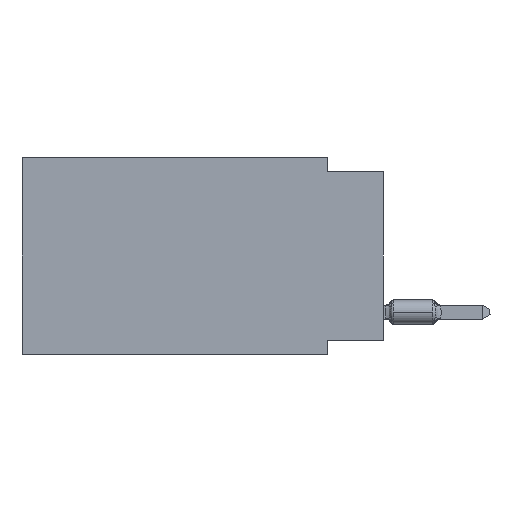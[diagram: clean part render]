
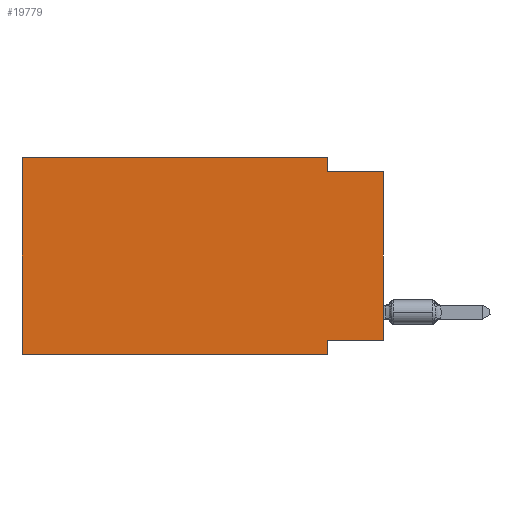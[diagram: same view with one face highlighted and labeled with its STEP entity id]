
A CAD part, left-side view. The second image highlights one B-rep face of the part: STEP entity #19779.
In plain terms, the highlighted planar face has unit normal (-1, 0, 0).
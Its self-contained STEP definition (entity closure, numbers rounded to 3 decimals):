
#254 = CARTESIAN_POINT ( 'NONE',  ( 0., 0., -0.635 ) ) ;
#355 = PLANE ( 'NONE',  #38991 ) ;
#422 = EDGE_CURVE ( 'NONE', #14213, #34933, #4034, .T. ) ;
#1116 = ORIENTED_EDGE ( 'NONE', *, *, #2686, .T. ) ;
#1243 = VECTOR ( 'NONE', #6488, 1000. ) ;
#1338 = EDGE_CURVE ( 'NONE', #21616, #13241, #23218, .T. ) ;
#1912 = VECTOR ( 'NONE', #14163, 1000. ) ;
#2667 = CARTESIAN_POINT ( 'NONE',  ( 0., 16.383, 0. ) ) ;
#2686 = EDGE_CURVE ( 'NONE', #12465, #34933, #25585, .T. ) ;
#2728 = EDGE_CURVE ( 'NONE', #37874, #23159, #19021, .T. ) ;
#4034 = LINE ( 'NONE', #16562, #15554 ) ;
#4400 = VECTOR ( 'NONE', #24400, 1000. ) ;
#6178 = LINE ( 'NONE', #14835, #15073 ) ;
#6387 = VECTOR ( 'NONE', #35505, 1000. ) ;
#6488 = DIRECTION ( 'NONE',  ( 0., -1., 0. ) ) ;
#8874 = VERTEX_POINT ( 'NONE', #24591 ) ;
#11290 = LINE ( 'NONE', #35510, #1912 ) ;
#11969 = CARTESIAN_POINT ( 'NONE',  ( 0., 2.54, -8.89 ) ) ;
#12181 = ORIENTED_EDGE ( 'NONE', *, *, #24088, .F. ) ;
#12465 = VERTEX_POINT ( 'NONE', #28687 ) ;
#12561 = DIRECTION ( 'NONE',  ( 0., 0., 1. ) ) ;
#13241 = VERTEX_POINT ( 'NONE', #254 ) ;
#13793 = DIRECTION ( 'NONE',  ( 0., 0., 1. ) ) ;
#14163 = DIRECTION ( 'NONE',  ( 0., -1., 0. ) ) ;
#14185 = CARTESIAN_POINT ( 'NONE',  ( 0., 0., 0. ) ) ;
#14213 = VERTEX_POINT ( 'NONE', #31699 ) ;
#14275 = ORIENTED_EDGE ( 'NONE', *, *, #422, .F. ) ;
#14835 = CARTESIAN_POINT ( 'NONE',  ( 0., 16.383, 0. ) ) ;
#15073 = VECTOR ( 'NONE', #12561, 1000. ) ;
#15554 = VECTOR ( 'NONE', #29067, 1000. ) ;
#16562 = CARTESIAN_POINT ( 'NONE',  ( 0., 2.54, -8.89 ) ) ;
#16997 = EDGE_LOOP ( 'NONE', ( #19865, #19341, #22470, #30613, #12181, #1116, #14275, #30127 ) ) ;
#19021 = LINE ( 'NONE', #22300, #33345 ) ;
#19050 = DIRECTION ( 'NONE',  ( 1., 0., 0. ) ) ;
#19341 = ORIENTED_EDGE ( 'NONE', *, *, #37628, .F. ) ;
#19422 = DIRECTION ( 'NONE',  ( 0., 0., -1. ) ) ;
#19779 = ADVANCED_FACE ( 'NONE', ( #22519 ), #355, .F. ) ;
#19865 = ORIENTED_EDGE ( 'NONE', *, *, #1338, .T. ) ;
#21616 = VERTEX_POINT ( 'NONE', #32470 ) ;
#22300 = CARTESIAN_POINT ( 'NONE',  ( 0., 2.54, 0. ) ) ;
#22470 = ORIENTED_EDGE ( 'NONE', *, *, #2728, .F. ) ;
#22519 = FACE_OUTER_BOUND ( 'NONE', #16997, .T. ) ;
#23001 = CARTESIAN_POINT ( 'NONE',  ( 0., 0., -0.635 ) ) ;
#23138 = EDGE_CURVE ( 'NONE', #8874, #37874, #11290, .T. ) ;
#23159 = VERTEX_POINT ( 'NONE', #26682 ) ;
#23218 = LINE ( 'NONE', #14185, #30099 ) ;
#24088 = EDGE_CURVE ( 'NONE', #12465, #8874, #6178, .T. ) ;
#24214 = LINE ( 'NONE', #36730, #4400 ) ;
#24400 = DIRECTION ( 'NONE',  ( 0., 1., 0. ) ) ;
#24591 = CARTESIAN_POINT ( 'NONE',  ( 0., 16.383, 0. ) ) ;
#24998 = CARTESIAN_POINT ( 'NONE',  ( 0., 2.54, 0. ) ) ;
#25155 = CARTESIAN_POINT ( 'NONE',  ( 0., 16.383, -8.89 ) ) ;
#25403 = DIRECTION ( 'NONE',  ( 0., 0., -1. ) ) ;
#25585 = LINE ( 'NONE', #25155, #1243 ) ;
#26682 = CARTESIAN_POINT ( 'NONE',  ( 0., 2.54, -0.635 ) ) ;
#28687 = CARTESIAN_POINT ( 'NONE',  ( 0., 16.383, -8.89 ) ) ;
#29067 = DIRECTION ( 'NONE',  ( 0., 0., -1. ) ) ;
#30099 = VECTOR ( 'NONE', #13793, 1000. ) ;
#30127 = ORIENTED_EDGE ( 'NONE', *, *, #37812, .F. ) ;
#30613 = ORIENTED_EDGE ( 'NONE', *, *, #23138, .F. ) ;
#31699 = CARTESIAN_POINT ( 'NONE',  ( 0., 2.54, -8.255 ) ) ;
#32470 = CARTESIAN_POINT ( 'NONE',  ( 0., 0., -8.255 ) ) ;
#33345 = VECTOR ( 'NONE', #19422, 1000. ) ;
#34933 = VERTEX_POINT ( 'NONE', #11969 ) ;
#35505 = DIRECTION ( 'NONE',  ( 0., -1., 0. ) ) ;
#35510 = CARTESIAN_POINT ( 'NONE',  ( 0., 16.383, 0. ) ) ;
#36730 = CARTESIAN_POINT ( 'NONE',  ( 0., 0., -8.255 ) ) ;
#37628 = EDGE_CURVE ( 'NONE', #23159, #13241, #38598, .T. ) ;
#37812 = EDGE_CURVE ( 'NONE', #21616, #14213, #24214, .T. ) ;
#37874 = VERTEX_POINT ( 'NONE', #24998 ) ;
#38598 = LINE ( 'NONE', #23001, #6387 ) ;
#38991 = AXIS2_PLACEMENT_3D ( 'NONE', #2667, #19050, #25403 ) ;
